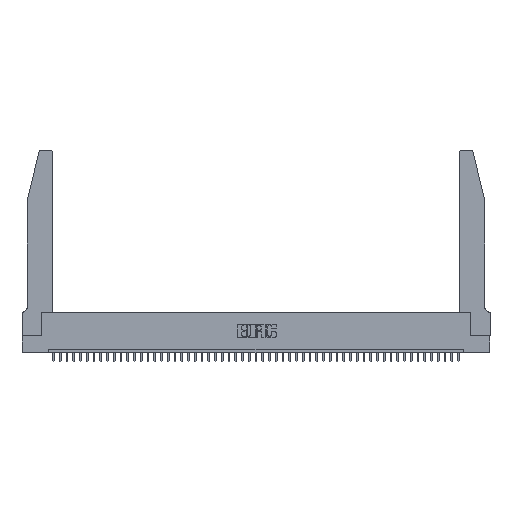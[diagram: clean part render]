
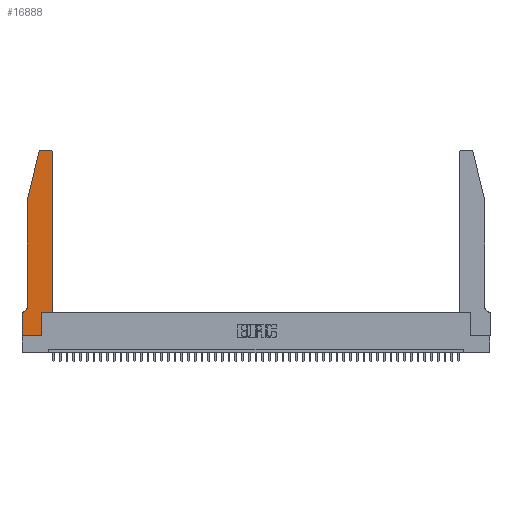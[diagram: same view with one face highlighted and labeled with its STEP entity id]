
A CAD part, top view. The second image highlights one B-rep face of the part: STEP entity #16888.
In plain terms, the highlighted planar face has unit normal (0, 0, 1).
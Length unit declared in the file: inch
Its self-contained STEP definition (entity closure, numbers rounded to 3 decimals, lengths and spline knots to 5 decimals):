
#892 = AXIS2_PLACEMENT_3D ( 'NONE', #25961, #14461, #19770 ) ;
#1294 = DIRECTION ( 'NONE',  ( 0., 0., -1. ) ) ;
#2701 = EDGE_CURVE ( 'NONE', #21203, #24612, #44807, .T. ) ;
#2727 = CARTESIAN_POINT ( 'NONE',  ( 0.0755, 2., 0.37 ) ) ;
#2861 = ORIENTED_EDGE ( 'NONE', *, *, #30554, .T. ) ;
#2980 = LINE ( 'NONE', #45748, #16896 ) ;
#2982 = EDGE_CURVE ( 'NONE', #31766, #15065, #37312, .T. ) ;
#3627 = VECTOR ( 'NONE', #6532, 39.37008 ) ;
#4076 = EDGE_CURVE ( 'NONE', #15065, #21203, #29635, .T. ) ;
#4355 = DIRECTION ( 'NONE',  ( 1., 0., 0. ) ) ;
#5320 = LINE ( 'NONE', #32184, #14622 ) ;
#6147 = CARTESIAN_POINT ( 'NONE',  ( 0.0755, 2., 0.37 ) ) ;
#6216 = LINE ( 'NONE', #24338, #10310 ) ;
#6444 = DIRECTION ( 'NONE',  ( 0., -1., 0. ) ) ;
#6532 = DIRECTION ( 'NONE',  ( 0., 1., 0. ) ) ;
#6873 = CARTESIAN_POINT ( 'NONE',  ( 0.25487, 2.72718, 0.37 ) ) ;
#7071 = VECTOR ( 'NONE', #6444, 39.37008 ) ;
#7603 = LINE ( 'NONE', #2727, #7071 ) ;
#8324 = DIRECTION ( 'NONE',  ( -1., 0., 0. ) ) ;
#9051 = DIRECTION ( 'NONE',  ( 1., 0., 0. ) ) ;
#9914 = DIRECTION ( 'NONE',  ( 0., 1., 0. ) ) ;
#10157 = EDGE_CURVE ( 'NONE', #43334, #17430, #39557, .T. ) ;
#10243 = DIRECTION ( 'NONE',  ( -0.239, -0.971, 0. ) ) ;
#10310 = VECTOR ( 'NONE', #9914, 39.37008 ) ;
#10311 = VECTOR ( 'NONE', #39103, 39.37008 ) ;
#11021 = EDGE_CURVE ( 'NONE', #24612, #43334, #47523, .T. ) ;
#11136 = ORIENTED_EDGE ( 'NONE', *, *, #11021, .T. ) ;
#13788 = LINE ( 'NONE', #20925, #10311 ) ;
#14083 = CARTESIAN_POINT ( 'NONE',  ( 0.0755, 0.42, 0.37 ) ) ;
#14461 = DIRECTION ( 'NONE',  ( 0., 0., 1. ) ) ;
#14622 = VECTOR ( 'NONE', #28756, 39.37008 ) ;
#15065 = VERTEX_POINT ( 'NONE', #44385 ) ;
#15678 = CARTESIAN_POINT ( 'NONE',  ( 0.0055, 0.35, 0.37 ) ) ;
#16123 = VERTEX_POINT ( 'NONE', #14083 ) ;
#16672 = VERTEX_POINT ( 'NONE', #25183 ) ;
#16888 = ADVANCED_FACE ( 'NONE', ( #19003 ), #28884, .T. ) ;
#16896 = VECTOR ( 'NONE', #4355, 39.37008 ) ;
#17294 = EDGE_CURVE ( 'NONE', #21846, #41958, #6216, .T. ) ;
#17430 = VERTEX_POINT ( 'NONE', #40698 ) ;
#17684 = ORIENTED_EDGE ( 'NONE', *, *, #27129, .T. ) ;
#17765 = CARTESIAN_POINT ( 'NONE',  ( 0.4505, 0.35, 0.37 ) ) ;
#19003 = FACE_OUTER_BOUND ( 'NONE', #19566, .T. ) ;
#19566 = EDGE_LOOP ( 'NONE', ( #36702, #11136, #37428, #32034, #17684, #23792, #2861, #46524, #40891, #31503, #47141, #19706 ) ) ;
#19657 = DIRECTION ( 'NONE',  ( -1., 0., 0. ) ) ;
#19706 = ORIENTED_EDGE ( 'NONE', *, *, #4076, .T. ) ;
#19770 = DIRECTION ( 'NONE',  ( 1., 0., 0. ) ) ;
#20098 = DIRECTION ( 'NONE',  ( 0., 0., 1. ) ) ;
#20132 = CARTESIAN_POINT ( 'NONE',  ( 0.4205, 2.75, 0.37 ) ) ;
#20177 = EDGE_CURVE ( 'NONE', #41958, #31766, #5320, .T. ) ;
#20612 = EDGE_CURVE ( 'NONE', #16672, #21846, #2980, .T. ) ;
#20810 = CARTESIAN_POINT ( 'NONE',  ( 0.284, 2.72, 0.37 ) ) ;
#20925 = CARTESIAN_POINT ( 'NONE',  ( 0.0755, 0.35, 0.37 ) ) ;
#21203 = VERTEX_POINT ( 'NONE', #20132 ) ;
#21846 = VERTEX_POINT ( 'NONE', #29461 ) ;
#23792 = ORIENTED_EDGE ( 'NONE', *, *, #40284, .T. ) ;
#24338 = CARTESIAN_POINT ( 'NONE',  ( 0.2865, 0.35, 0.37 ) ) ;
#24612 = VERTEX_POINT ( 'NONE', #43469 ) ;
#25183 = CARTESIAN_POINT ( 'NONE',  ( 0., 0., 0.37 ) ) ;
#25961 = CARTESIAN_POINT ( 'NONE',  ( 0., 0.35, 0.37 ) ) ;
#26642 = CARTESIAN_POINT ( 'NONE',  ( 0., 0., 0.37 ) ) ;
#27129 = EDGE_CURVE ( 'NONE', #16123, #28768, #34931, .T. ) ;
#28417 = CARTESIAN_POINT ( 'NONE',  ( 0.2865, 0.35, 0.37 ) ) ;
#28756 = DIRECTION ( 'NONE',  ( 1., 0., 0. ) ) ;
#28768 = VERTEX_POINT ( 'NONE', #15678 ) ;
#28884 = PLANE ( 'NONE',  #892 ) ;
#29461 = CARTESIAN_POINT ( 'NONE',  ( 0.2865, 0., 0.37 ) ) ;
#29635 = CIRCLE ( 'NONE', #37779, 0.03 ) ;
#29921 = VERTEX_POINT ( 'NONE', #45485 ) ;
#30554 = EDGE_CURVE ( 'NONE', #29921, #16672, #45904, .T. ) ;
#30787 = CARTESIAN_POINT ( 'NONE',  ( 0.4205, 2.72, 0.37 ) ) ;
#31089 = CARTESIAN_POINT ( 'NONE',  ( 0.2605, 2.75, 0.37 ) ) ;
#31503 = ORIENTED_EDGE ( 'NONE', *, *, #20177, .T. ) ;
#31766 = VERTEX_POINT ( 'NONE', #33172 ) ;
#32034 = ORIENTED_EDGE ( 'NONE', *, *, #47623, .T. ) ;
#32184 = CARTESIAN_POINT ( 'NONE',  ( 0.4505, 0.35, 0.37 ) ) ;
#33172 = CARTESIAN_POINT ( 'NONE',  ( 0.4505, 0.35, 0.37 ) ) ;
#33829 = DIRECTION ( 'NONE',  ( 0., -1., 0. ) ) ;
#34931 = CIRCLE ( 'NONE', #43576, 0.07 ) ;
#35104 = CARTESIAN_POINT ( 'NONE',  ( 0.0055, 0.42, 0.37 ) ) ;
#35436 = DIRECTION ( 'NONE',  ( 1., 0., 0. ) ) ;
#36702 = ORIENTED_EDGE ( 'NONE', *, *, #2701, .T. ) ;
#37210 = VECTOR ( 'NONE', #10243, 39.37008 ) ;
#37312 = LINE ( 'NONE', #17765, #3627 ) ;
#37428 = ORIENTED_EDGE ( 'NONE', *, *, #10157, .T. ) ;
#37779 = AXIS2_PLACEMENT_3D ( 'NONE', #30787, #20098, #9051 ) ;
#38387 = VECTOR ( 'NONE', #33829, 39.37008 ) ;
#39103 = DIRECTION ( 'NONE',  ( -1., 0., 0. ) ) ;
#39557 = LINE ( 'NONE', #6147, #37210 ) ;
#40284 = EDGE_CURVE ( 'NONE', #28768, #29921, #13788, .T. ) ;
#40698 = CARTESIAN_POINT ( 'NONE',  ( 0.0755, 2., 0.37 ) ) ;
#40811 = VECTOR ( 'NONE', #8324, 39.37008 ) ;
#40891 = ORIENTED_EDGE ( 'NONE', *, *, #17294, .T. ) ;
#41958 = VERTEX_POINT ( 'NONE', #28417 ) ;
#43334 = VERTEX_POINT ( 'NONE', #6873 ) ;
#43469 = CARTESIAN_POINT ( 'NONE',  ( 0.284, 2.75, 0.37 ) ) ;
#43576 = AXIS2_PLACEMENT_3D ( 'NONE', #35104, #1294, #19657 ) ;
#44385 = CARTESIAN_POINT ( 'NONE',  ( 0.4505, 2.72, 0.37 ) ) ;
#44807 = LINE ( 'NONE', #31089, #40811 ) ;
#45485 = CARTESIAN_POINT ( 'NONE',  ( 0., 0.35, 0.37 ) ) ;
#45748 = CARTESIAN_POINT ( 'NONE',  ( 0., 0., 0.37 ) ) ;
#45904 = LINE ( 'NONE', #26642, #38387 ) ;
#46524 = ORIENTED_EDGE ( 'NONE', *, *, #20612, .T. ) ;
#47082 = DIRECTION ( 'NONE',  ( 0., 0., 1. ) ) ;
#47141 = ORIENTED_EDGE ( 'NONE', *, *, #2982, .T. ) ;
#47465 = AXIS2_PLACEMENT_3D ( 'NONE', #20810, #47082, #35436 ) ;
#47523 = CIRCLE ( 'NONE', #47465, 0.03 ) ;
#47623 = EDGE_CURVE ( 'NONE', #17430, #16123, #7603, .T. ) ;
